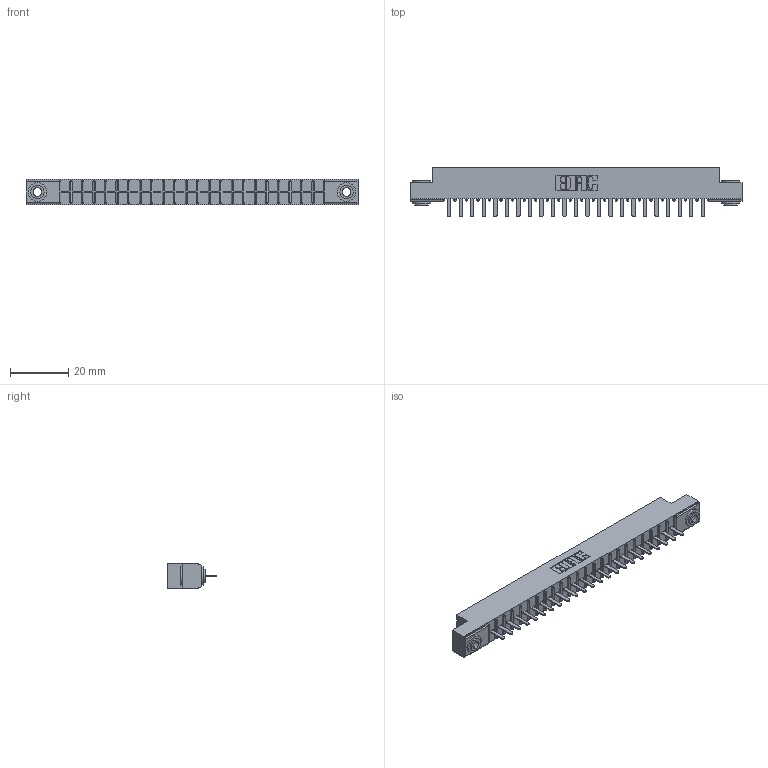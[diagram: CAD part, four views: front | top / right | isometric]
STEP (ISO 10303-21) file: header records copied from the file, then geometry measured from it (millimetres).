
FILE_DESCRIPTION (( 'STEP AP203' ), '1' );
FILE_NAME ('356-023-420-103.STEP', '2020-09-23T15:51:26', ( '' ), ( '' ), 'SwSTEP 2.0', 'SolidWorks 2020', '' );
FILE_SCHEMA (( 'CONFIG_CONTROL_DESIGN' ));
Length unit declared in the file: inch
Products named in the file (4): 306 Part_.156 Dia; 345-250-002_345-250-002-102; 356-023-420-103; 306-290-001_120
Assembly tree (26 placements, depth 2):
  356-023-420-103
    306 Part_.156 Dia
    306-290-001_120  x23
    345-250-002_345-250-002-102  x2
Bounding box: 114.15 x 17.12 x 8.71 mm (x, y, z)
Volume: 7811.8 mm3; surface area: 11845.9 mm2
Topology: 26 solids, 26 shells, 1778 faces, 4959 edges, 3178 vertices
Faces by surface type: plane 1173, cylinder 505, sphere 92, cone 8
Entity records: 24931 total; most frequent: CARTESIAN_POINT 4161, DIRECTION 4119, ORIENTED_EDGE 4114, EDGE_CURVE 2057, VECTOR 1591, LINE 1591, VERTEX_POINT 1306, AXIS2_PLACEMENT_3D 1264
